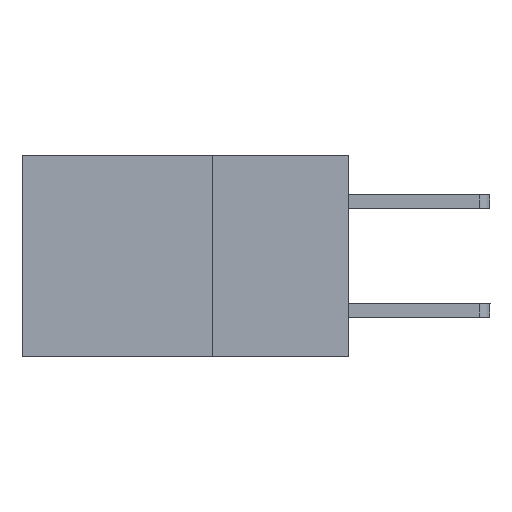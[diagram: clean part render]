
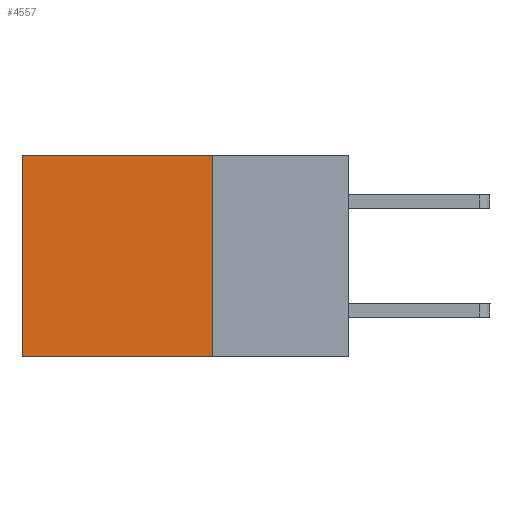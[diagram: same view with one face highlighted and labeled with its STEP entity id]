
A CAD part, left-side view. The second image highlights one B-rep face of the part: STEP entity #4557.
In plain terms, the highlighted planar face has unit normal (-1, 0, 0).
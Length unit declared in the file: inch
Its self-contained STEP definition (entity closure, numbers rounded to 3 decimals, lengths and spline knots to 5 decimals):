
#105 = VERTEX_POINT ( 'NONE', #7978 ) ;
#845 = DIRECTION ( 'NONE',  ( 0., 0., -1. ) ) ;
#859 = ORIENTED_EDGE ( 'NONE', *, *, #9276, .F. ) ;
#1307 = VERTEX_POINT ( 'NONE', #2899 ) ;
#2307 = VECTOR ( 'NONE', #4496, 39.37008 ) ;
#2368 = EDGE_CURVE ( 'NONE', #105, #5162, #9278, .T. ) ;
#2539 = EDGE_CURVE ( 'NONE', #1307, #6705, #4051, .T. ) ;
#2573 = CARTESIAN_POINT ( 'NONE',  ( 0.2615, 0.6, -0.37 ) ) ;
#2838 = CARTESIAN_POINT ( 'NONE',  ( 0.2615, 0.25, -0.37 ) ) ;
#2899 = CARTESIAN_POINT ( 'NONE',  ( 0.2615, 0.25, 0. ) ) ;
#3712 = DIRECTION ( 'NONE',  ( 0., 0., -1. ) ) ;
#4051 = LINE ( 'NONE', #5734, #2307 ) ;
#4246 = DIRECTION ( 'NONE',  ( 1., 0., 0. ) ) ;
#4257 = PLANE ( 'NONE',  #9132 ) ;
#4268 = LINE ( 'NONE', #8817, #5785 ) ;
#4455 = CARTESIAN_POINT ( 'NONE',  ( 0.2615, 0.6, 0. ) ) ;
#4496 = DIRECTION ( 'NONE',  ( 0., 1., 0. ) ) ;
#4557 = ADVANCED_FACE ( 'NONE', ( #6358 ), #4257, .F. ) ;
#4807 = ORIENTED_EDGE ( 'NONE', *, *, #7747, .T. ) ;
#4827 = LINE ( 'NONE', #5307, #8694 ) ;
#5162 = VERTEX_POINT ( 'NONE', #2573 ) ;
#5307 = CARTESIAN_POINT ( 'NONE',  ( 0.2615, 0.25, -0.37 ) ) ;
#5709 = ORIENTED_EDGE ( 'NONE', *, *, #2368, .F. ) ;
#5734 = CARTESIAN_POINT ( 'NONE',  ( 0.2615, 0.25, 0. ) ) ;
#5785 = VECTOR ( 'NONE', #3712, 39.37008 ) ;
#6130 = EDGE_LOOP ( 'NONE', ( #4807, #5709, #859, #8169 ) ) ;
#6179 = CARTESIAN_POINT ( 'NONE',  ( 0.2615, 0.25, -0.37 ) ) ;
#6358 = FACE_OUTER_BOUND ( 'NONE', #6130, .T. ) ;
#6705 = VERTEX_POINT ( 'NONE', #4455 ) ;
#6866 = DIRECTION ( 'NONE',  ( 0., 1., 0. ) ) ;
#7482 = DIRECTION ( 'NONE',  ( 0., 0., -1. ) ) ;
#7747 = EDGE_CURVE ( 'NONE', #6705, #5162, #4268, .T. ) ;
#7861 = VECTOR ( 'NONE', #6866, 39.37008 ) ;
#7978 = CARTESIAN_POINT ( 'NONE',  ( 0.2615, 0.25, -0.37 ) ) ;
#8169 = ORIENTED_EDGE ( 'NONE', *, *, #2539, .T. ) ;
#8694 = VECTOR ( 'NONE', #845, 39.37008 ) ;
#8817 = CARTESIAN_POINT ( 'NONE',  ( 0.2615, 0.6, -0.37 ) ) ;
#9132 = AXIS2_PLACEMENT_3D ( 'NONE', #2838, #4246, #7482 ) ;
#9276 = EDGE_CURVE ( 'NONE', #1307, #105, #4827, .T. ) ;
#9278 = LINE ( 'NONE', #6179, #7861 ) ;
